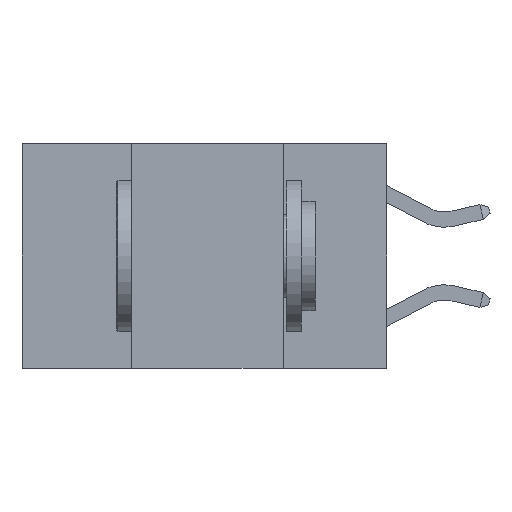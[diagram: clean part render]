
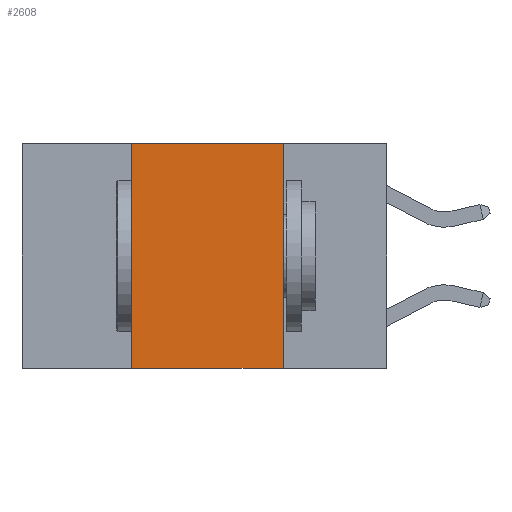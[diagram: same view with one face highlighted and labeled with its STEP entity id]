
A CAD part, left-side view. The second image highlights one B-rep face of the part: STEP entity #2608.
In plain terms, the highlighted planar face has unit normal (-1, 0, 0).
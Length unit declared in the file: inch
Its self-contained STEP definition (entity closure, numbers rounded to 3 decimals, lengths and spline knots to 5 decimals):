
#1088 = CARTESIAN_POINT ( 'NONE',  ( 0., 0.42, 0. ) ) ;
#1511 = VERTEX_POINT ( 'NONE', #12166 ) ;
#2155 = LINE ( 'NONE', #2914, #14119 ) ;
#2608 = ADVANCED_FACE ( 'NONE', ( #9349 ), #11653, .F. ) ;
#2914 = CARTESIAN_POINT ( 'NONE',  ( 0., 0.17, 0. ) ) ;
#3004 = DIRECTION ( 'NONE',  ( 0., 0., 1. ) ) ;
#3520 = CARTESIAN_POINT ( 'NONE',  ( 0., 0.17, 0. ) ) ;
#3680 = CARTESIAN_POINT ( 'NONE',  ( 0., 0.6, 0. ) ) ;
#3952 = EDGE_LOOP ( 'NONE', ( #4483, #6153, #7208, #6622 ) ) ;
#4483 = ORIENTED_EDGE ( 'NONE', *, *, #5813, .F. ) ;
#5813 = EDGE_CURVE ( 'NONE', #12214, #6988, #2155, .T. ) ;
#6153 = ORIENTED_EDGE ( 'NONE', *, *, #13308, .F. ) ;
#6622 = ORIENTED_EDGE ( 'NONE', *, *, #14322, .T. ) ;
#6719 = EDGE_CURVE ( 'NONE', #1511, #10106, #12195, .T. ) ;
#6988 = VERTEX_POINT ( 'NONE', #7376 ) ;
#7208 = ORIENTED_EDGE ( 'NONE', *, *, #6719, .F. ) ;
#7376 = CARTESIAN_POINT ( 'NONE',  ( 0., 0.17, -0.37 ) ) ;
#7604 = DIRECTION ( 'NONE',  ( 0., -1., 0. ) ) ;
#7612 = VECTOR ( 'NONE', #7604, 39.37008 ) ;
#7689 = CARTESIAN_POINT ( 'NONE',  ( 0., 0.42, 0. ) ) ;
#7920 = LINE ( 'NONE', #10024, #7612 ) ;
#8268 = DIRECTION ( 'NONE',  ( 1., 0., 0. ) ) ;
#8436 = VECTOR ( 'NONE', #3004, 39.37008 ) ;
#8568 = DIRECTION ( 'NONE',  ( 0., -1., 0. ) ) ;
#9116 = AXIS2_PLACEMENT_3D ( 'NONE', #3680, #8268, #12858 ) ;
#9349 = FACE_OUTER_BOUND ( 'NONE', #3952, .T. ) ;
#9643 = LINE ( 'NONE', #12025, #13410 ) ;
#10024 = CARTESIAN_POINT ( 'NONE',  ( 0., 0.6, -0.37 ) ) ;
#10106 = VERTEX_POINT ( 'NONE', #1088 ) ;
#11653 = PLANE ( 'NONE',  #9116 ) ;
#12025 = CARTESIAN_POINT ( 'NONE',  ( 0., 0.6, 0. ) ) ;
#12166 = CARTESIAN_POINT ( 'NONE',  ( 0., 0.42, -0.37 ) ) ;
#12195 = LINE ( 'NONE', #7689, #8436 ) ;
#12214 = VERTEX_POINT ( 'NONE', #3520 ) ;
#12858 = DIRECTION ( 'NONE',  ( 0., 0., -1. ) ) ;
#13308 = EDGE_CURVE ( 'NONE', #10106, #12214, #9643, .T. ) ;
#13317 = DIRECTION ( 'NONE',  ( 0., 0., -1. ) ) ;
#13410 = VECTOR ( 'NONE', #8568, 39.37008 ) ;
#14119 = VECTOR ( 'NONE', #13317, 39.37008 ) ;
#14322 = EDGE_CURVE ( 'NONE', #1511, #6988, #7920, .T. ) ;
